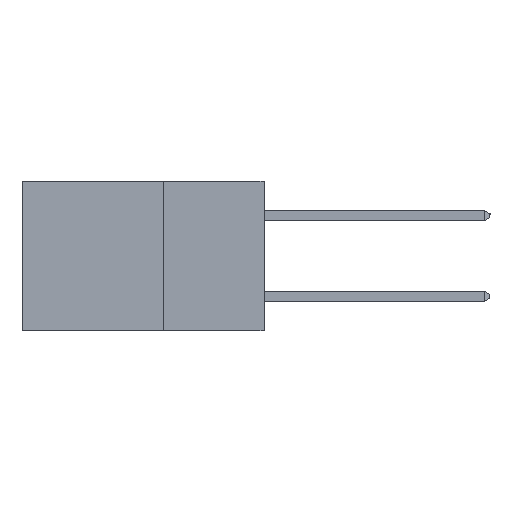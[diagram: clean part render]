
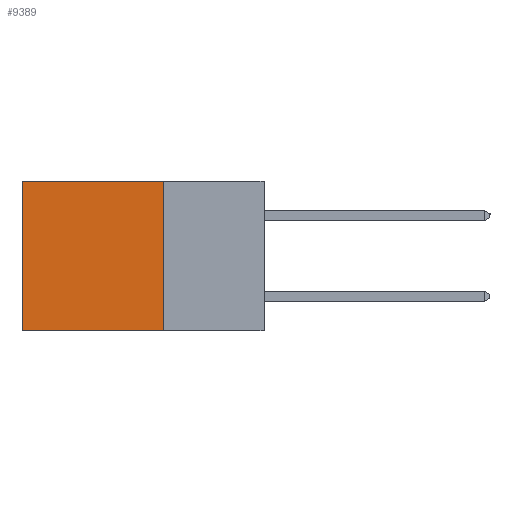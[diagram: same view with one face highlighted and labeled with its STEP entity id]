
A CAD part, left-side view. The second image highlights one B-rep face of the part: STEP entity #9389.
In plain terms, the highlighted planar face has unit normal (-1, 0, 0).
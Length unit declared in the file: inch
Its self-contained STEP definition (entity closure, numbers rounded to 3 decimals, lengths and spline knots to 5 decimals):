
#692 = LINE ( 'NONE', #1514, #8215 ) ;
#795 = LINE ( 'NONE', #5034, #11526 ) ;
#1514 = CARTESIAN_POINT ( 'NONE',  ( 0.2615, 0.6, -0.37 ) ) ;
#2091 = DIRECTION ( 'NONE',  ( 1., 0., 0. ) ) ;
#2098 = EDGE_CURVE ( 'NONE', #4087, #8220, #6623, .T. ) ;
#2559 = EDGE_LOOP ( 'NONE', ( #11075, #11936, #11967, #7908 ) ) ;
#2937 = VERTEX_POINT ( 'NONE', #4924 ) ;
#4087 = VERTEX_POINT ( 'NONE', #7562 ) ;
#4509 = VECTOR ( 'NONE', #11747, 39.37008 ) ;
#4780 = DIRECTION ( 'NONE',  ( 0., 1., 0. ) ) ;
#4924 = CARTESIAN_POINT ( 'NONE',  ( 0.2615, 0.25, -0.37 ) ) ;
#5034 = CARTESIAN_POINT ( 'NONE',  ( 0.2615, 0.25, -0.37 ) ) ;
#6328 = PLANE ( 'NONE',  #9500 ) ;
#6623 = LINE ( 'NONE', #10846, #4509 ) ;
#6647 = CARTESIAN_POINT ( 'NONE',  ( 0.2615, 0.6, -0.37 ) ) ;
#6959 = EDGE_CURVE ( 'NONE', #2937, #8584, #11283, .T. ) ;
#7111 = DIRECTION ( 'NONE',  ( 0., 0., -1. ) ) ;
#7548 = EDGE_CURVE ( 'NONE', #4087, #2937, #795, .T. ) ;
#7562 = CARTESIAN_POINT ( 'NONE',  ( 0.2615, 0.25, 0. ) ) ;
#7830 = CARTESIAN_POINT ( 'NONE',  ( 0.2615, 0.6, 0. ) ) ;
#7908 = ORIENTED_EDGE ( 'NONE', *, *, #2098, .T. ) ;
#8215 = VECTOR ( 'NONE', #11287, 39.37008 ) ;
#8220 = VERTEX_POINT ( 'NONE', #7830 ) ;
#8275 = EDGE_CURVE ( 'NONE', #8220, #8584, #692, .T. ) ;
#8584 = VERTEX_POINT ( 'NONE', #6647 ) ;
#8997 = CARTESIAN_POINT ( 'NONE',  ( 0.2615, 0.25, -0.37 ) ) ;
#9389 = ADVANCED_FACE ( 'NONE', ( #12781 ), #6328, .F. ) ;
#9500 = AXIS2_PLACEMENT_3D ( 'NONE', #11595, #2091, #10751 ) ;
#10751 = DIRECTION ( 'NONE',  ( 0., 0., -1. ) ) ;
#10846 = CARTESIAN_POINT ( 'NONE',  ( 0.2615, 0.25, 0. ) ) ;
#11075 = ORIENTED_EDGE ( 'NONE', *, *, #8275, .T. ) ;
#11283 = LINE ( 'NONE', #8997, #11314 ) ;
#11287 = DIRECTION ( 'NONE',  ( 0., 0., -1. ) ) ;
#11314 = VECTOR ( 'NONE', #4780, 39.37008 ) ;
#11526 = VECTOR ( 'NONE', #7111, 39.37008 ) ;
#11595 = CARTESIAN_POINT ( 'NONE',  ( 0.2615, 0.25, -0.37 ) ) ;
#11747 = DIRECTION ( 'NONE',  ( 0., 1., 0. ) ) ;
#11936 = ORIENTED_EDGE ( 'NONE', *, *, #6959, .F. ) ;
#11967 = ORIENTED_EDGE ( 'NONE', *, *, #7548, .F. ) ;
#12781 = FACE_OUTER_BOUND ( 'NONE', #2559, .T. ) ;
